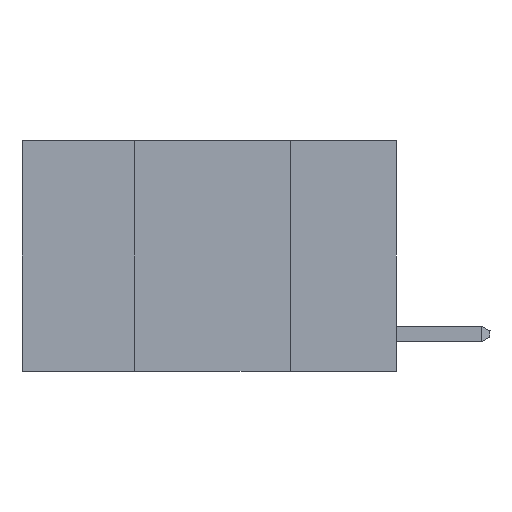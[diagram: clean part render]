
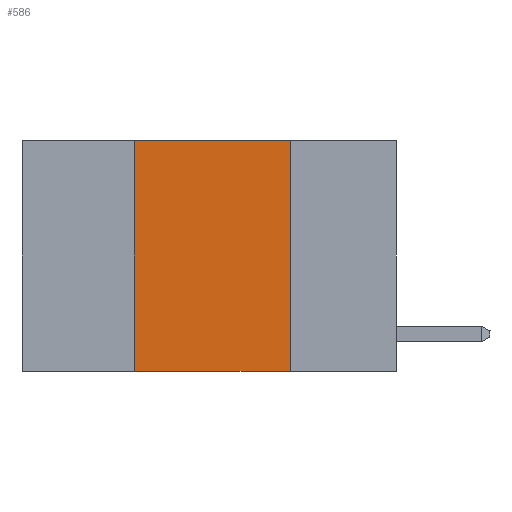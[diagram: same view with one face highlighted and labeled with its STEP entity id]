
A CAD part, left-side view. The second image highlights one B-rep face of the part: STEP entity #586.
In plain terms, the highlighted planar face has unit normal (-1, 0, 0).
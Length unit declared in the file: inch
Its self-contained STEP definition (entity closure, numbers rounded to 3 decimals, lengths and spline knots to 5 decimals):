
#586 = ADVANCED_FACE ( 'NONE', ( #17228 ), #792, .F. ) ;
#792 = PLANE ( 'NONE',  #17626 ) ;
#2447 = ORIENTED_EDGE ( 'NONE', *, *, #3512, .F. ) ;
#3512 = EDGE_CURVE ( 'NONE', #7461, #12720, #14564, .T. ) ;
#4829 = LINE ( 'NONE', #17520, #11857 ) ;
#5180 = DIRECTION ( 'NONE',  ( 0., 0., -1. ) ) ;
#5450 = VECTOR ( 'NONE', #8616, 39.37008 ) ;
#6584 = ORIENTED_EDGE ( 'NONE', *, *, #20373, .F. ) ;
#7461 = VERTEX_POINT ( 'NONE', #8195 ) ;
#7887 = VECTOR ( 'NONE', #15977, 39.37008 ) ;
#8195 = CARTESIAN_POINT ( 'NONE',  ( 0., 0.17, 0. ) ) ;
#8616 = DIRECTION ( 'NONE',  ( 0., -1., 0. ) ) ;
#9271 = DIRECTION ( 'NONE',  ( 0., 0., 1. ) ) ;
#9484 = DIRECTION ( 'NONE',  ( 0., 0., -1. ) ) ;
#10146 = VECTOR ( 'NONE', #5180, 39.37008 ) ;
#10652 = ORIENTED_EDGE ( 'NONE', *, *, #13732, .T. ) ;
#11009 = CARTESIAN_POINT ( 'NONE',  ( 0., 0.6, 0. ) ) ;
#11857 = VECTOR ( 'NONE', #9271, 39.37008 ) ;
#12497 = LINE ( 'NONE', #13045, #5450 ) ;
#12720 = VERTEX_POINT ( 'NONE', #20183 ) ;
#13045 = CARTESIAN_POINT ( 'NONE',  ( 0., 0.6, -0.37 ) ) ;
#13732 = EDGE_CURVE ( 'NONE', #17525, #12720, #12497, .T. ) ;
#14227 = ORIENTED_EDGE ( 'NONE', *, *, #17594, .F. ) ;
#14412 = LINE ( 'NONE', #11009, #7887 ) ;
#14564 = LINE ( 'NONE', #16745, #10146 ) ;
#15041 = EDGE_LOOP ( 'NONE', ( #2447, #14227, #6584, #10652 ) ) ;
#15845 = VERTEX_POINT ( 'NONE', #19443 ) ;
#15977 = DIRECTION ( 'NONE',  ( 0., -1., 0. ) ) ;
#16745 = CARTESIAN_POINT ( 'NONE',  ( 0., 0.17, 0. ) ) ;
#17228 = FACE_OUTER_BOUND ( 'NONE', #15041, .T. ) ;
#17520 = CARTESIAN_POINT ( 'NONE',  ( 0., 0.42, 0. ) ) ;
#17525 = VERTEX_POINT ( 'NONE', #20502 ) ;
#17594 = EDGE_CURVE ( 'NONE', #15845, #7461, #14412, .T. ) ;
#17626 = AXIS2_PLACEMENT_3D ( 'NONE', #17879, #19705, #9484 ) ;
#17879 = CARTESIAN_POINT ( 'NONE',  ( 0., 0.6, 0. ) ) ;
#19443 = CARTESIAN_POINT ( 'NONE',  ( 0., 0.42, 0. ) ) ;
#19705 = DIRECTION ( 'NONE',  ( 1., 0., 0. ) ) ;
#20183 = CARTESIAN_POINT ( 'NONE',  ( 0., 0.17, -0.37 ) ) ;
#20373 = EDGE_CURVE ( 'NONE', #17525, #15845, #4829, .T. ) ;
#20502 = CARTESIAN_POINT ( 'NONE',  ( 0., 0.42, -0.37 ) ) ;
